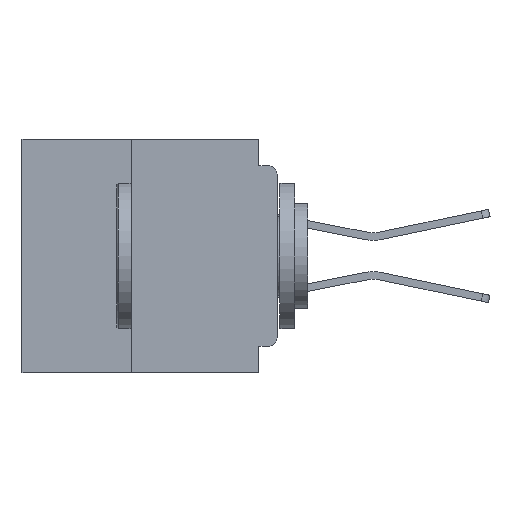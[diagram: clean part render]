
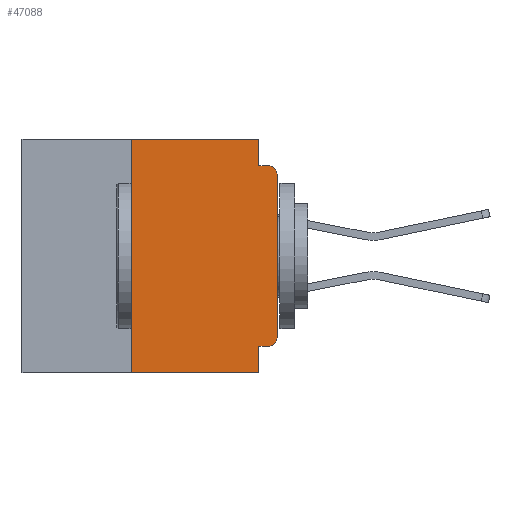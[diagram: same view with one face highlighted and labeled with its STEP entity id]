
A CAD part, left-side view. The second image highlights one B-rep face of the part: STEP entity #47088.
In plain terms, the highlighted planar face has unit normal (-1, 0, 0).
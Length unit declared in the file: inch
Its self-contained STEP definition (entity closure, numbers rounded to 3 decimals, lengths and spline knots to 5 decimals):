
#450 = ORIENTED_EDGE ( 'NONE', *, *, #30408, .F. ) ;
#862 = VECTOR ( 'NONE', #23540, 39.37008 ) ;
#1203 = CARTESIAN_POINT ( 'NONE',  ( 0., 0.015, -0.355 ) ) ;
#3593 = CARTESIAN_POINT ( 'NONE',  ( 0., 0.437, -0.4 ) ) ;
#3683 = DIRECTION ( 'NONE',  ( 0., 0., 1. ) ) ;
#3736 = LINE ( 'NONE', #29587, #23475 ) ;
#3756 = CARTESIAN_POINT ( 'NONE',  ( 0., 0.031, -0.045 ) ) ;
#3899 = ORIENTED_EDGE ( 'NONE', *, *, #17130, .F. ) ;
#4261 = VECTOR ( 'NONE', #12332, 39.37008 ) ;
#4723 = CARTESIAN_POINT ( 'NONE',  ( 0., 0.25, -0.4 ) ) ;
#5860 = LINE ( 'NONE', #29556, #34204 ) ;
#6867 = EDGE_LOOP ( 'NONE', ( #45768, #18925, #17181, #15475, #3899, #11438, #39293, #18139, #450, #16743 ) ) ;
#7602 = VERTEX_POINT ( 'NONE', #31154 ) ;
#8977 = EDGE_CURVE ( 'NONE', #7602, #32404, #32501, .T. ) ;
#11030 = CARTESIAN_POINT ( 'NONE',  ( 0., 0.015, -0.045 ) ) ;
#11438 = ORIENTED_EDGE ( 'NONE', *, *, #18230, .F. ) ;
#11637 = CIRCLE ( 'NONE', #36680, 0.015 ) ;
#11665 = VECTOR ( 'NONE', #13619, 39.37008 ) ;
#11963 = VECTOR ( 'NONE', #21723, 39.37008 ) ;
#12332 = DIRECTION ( 'NONE',  ( 0., -1., 0. ) ) ;
#13075 = AXIS2_PLACEMENT_3D ( 'NONE', #27691, #16707, #42415 ) ;
#13619 = DIRECTION ( 'NONE',  ( 0., 0., -1. ) ) ;
#14135 = LINE ( 'NONE', #19679, #4261 ) ;
#14350 = CARTESIAN_POINT ( 'NONE',  ( 0., 0.031, 0. ) ) ;
#14410 = LINE ( 'NONE', #3593, #32879 ) ;
#14747 = VERTEX_POINT ( 'NONE', #14350 ) ;
#15475 = ORIENTED_EDGE ( 'NONE', *, *, #26788, .F. ) ;
#15486 = EDGE_CURVE ( 'NONE', #46969, #32404, #14410, .T. ) ;
#15633 = VERTEX_POINT ( 'NONE', #3756 ) ;
#16208 = CARTESIAN_POINT ( 'NONE',  ( 0., 0.015, -0.34 ) ) ;
#16707 = DIRECTION ( 'NONE',  ( 1., 0., 0. ) ) ;
#16743 = ORIENTED_EDGE ( 'NONE', *, *, #18516, .T. ) ;
#17130 = EDGE_CURVE ( 'NONE', #38773, #14747, #14135, .T. ) ;
#17181 = ORIENTED_EDGE ( 'NONE', *, *, #41822, .F. ) ;
#18139 = ORIENTED_EDGE ( 'NONE', *, *, #8977, .F. ) ;
#18230 = EDGE_CURVE ( 'NONE', #46969, #38773, #5860, .T. ) ;
#18361 = DIRECTION ( 'NONE',  ( 0., -1., 0. ) ) ;
#18516 = EDGE_CURVE ( 'NONE', #42060, #45177, #11637, .T. ) ;
#18925 = ORIENTED_EDGE ( 'NONE', *, *, #33725, .T. ) ;
#19679 = CARTESIAN_POINT ( 'NONE',  ( 0., 0.437, 0. ) ) ;
#19722 = LINE ( 'NONE', #33254, #38066 ) ;
#19809 = CARTESIAN_POINT ( 'NONE',  ( 0., 0.031, 0. ) ) ;
#19947 = DIRECTION ( 'NONE',  ( 0., 0., -1. ) ) ;
#20692 = DIRECTION ( 'NONE',  ( -1., 0., 0. ) ) ;
#20944 = CARTESIAN_POINT ( 'NONE',  ( 0., 0.031, -0.4 ) ) ;
#21723 = DIRECTION ( 'NONE',  ( 0., 0., 1. ) ) ;
#21797 = LINE ( 'NONE', #19809, #862 ) ;
#21880 = LINE ( 'NONE', #36283, #11963 ) ;
#23475 = VECTOR ( 'NONE', #33273, 39.37008 ) ;
#23540 = DIRECTION ( 'NONE',  ( 0., 0., -1. ) ) ;
#23700 = CIRCLE ( 'NONE', #39726, 0.015 ) ;
#24209 = CARTESIAN_POINT ( 'NONE',  ( 0., 0., -0.34 ) ) ;
#26788 = EDGE_CURVE ( 'NONE', #14747, #15633, #21797, .T. ) ;
#27465 = VERTEX_POINT ( 'NONE', #11030 ) ;
#27691 = CARTESIAN_POINT ( 'NONE',  ( 0., 0.437, 0. ) ) ;
#29556 = CARTESIAN_POINT ( 'NONE',  ( 0., 0.25, -0.4 ) ) ;
#29587 = CARTESIAN_POINT ( 'NONE',  ( 0., 0., -0.355 ) ) ;
#29622 = CARTESIAN_POINT ( 'NONE',  ( 0., 0., -0.06 ) ) ;
#30408 = EDGE_CURVE ( 'NONE', #42060, #7602, #3736, .T. ) ;
#30590 = CARTESIAN_POINT ( 'NONE',  ( 0., 0.25, 0. ) ) ;
#31154 = CARTESIAN_POINT ( 'NONE',  ( 0., 0.031, -0.355 ) ) ;
#32404 = VERTEX_POINT ( 'NONE', #38186 ) ;
#32501 = LINE ( 'NONE', #20944, #11665 ) ;
#32879 = VECTOR ( 'NONE', #18361, 39.37008 ) ;
#33254 = CARTESIAN_POINT ( 'NONE',  ( 0., 0., -0.045 ) ) ;
#33273 = DIRECTION ( 'NONE',  ( 0., 1., 0. ) ) ;
#33725 = EDGE_CURVE ( 'NONE', #34625, #27465, #23700, .T. ) ;
#34204 = VECTOR ( 'NONE', #3683, 39.37008 ) ;
#34625 = VERTEX_POINT ( 'NONE', #29622 ) ;
#36283 = CARTESIAN_POINT ( 'NONE',  ( 0., 0., 0. ) ) ;
#36680 = AXIS2_PLACEMENT_3D ( 'NONE', #16208, #41893, #19947 ) ;
#36916 = DIRECTION ( 'NONE',  ( 0., -1., 0. ) ) ;
#38066 = VECTOR ( 'NONE', #36916, 39.37008 ) ;
#38179 = FACE_OUTER_BOUND ( 'NONE', #6867, .T. ) ;
#38186 = CARTESIAN_POINT ( 'NONE',  ( 0., 0.031, -0.4 ) ) ;
#38715 = PLANE ( 'NONE',  #13075 ) ;
#38773 = VERTEX_POINT ( 'NONE', #30590 ) ;
#39293 = ORIENTED_EDGE ( 'NONE', *, *, #15486, .T. ) ;
#39726 = AXIS2_PLACEMENT_3D ( 'NONE', #42629, #20692, #46276 ) ;
#41822 = EDGE_CURVE ( 'NONE', #15633, #27465, #19722, .T. ) ;
#41893 = DIRECTION ( 'NONE',  ( -1., 0., 0. ) ) ;
#42060 = VERTEX_POINT ( 'NONE', #1203 ) ;
#42415 = DIRECTION ( 'NONE',  ( 0., 0., -1. ) ) ;
#42629 = CARTESIAN_POINT ( 'NONE',  ( 0., 0.015, -0.06 ) ) ;
#43563 = EDGE_CURVE ( 'NONE', #45177, #34625, #21880, .T. ) ;
#45177 = VERTEX_POINT ( 'NONE', #24209 ) ;
#45768 = ORIENTED_EDGE ( 'NONE', *, *, #43563, .T. ) ;
#46276 = DIRECTION ( 'NONE',  ( 0., 0., -1. ) ) ;
#46969 = VERTEX_POINT ( 'NONE', #4723 ) ;
#47088 = ADVANCED_FACE ( 'NONE', ( #38179 ), #38715, .F. ) ;
